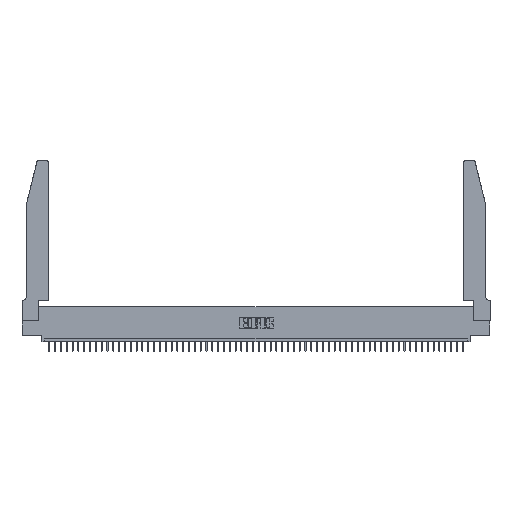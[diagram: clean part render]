
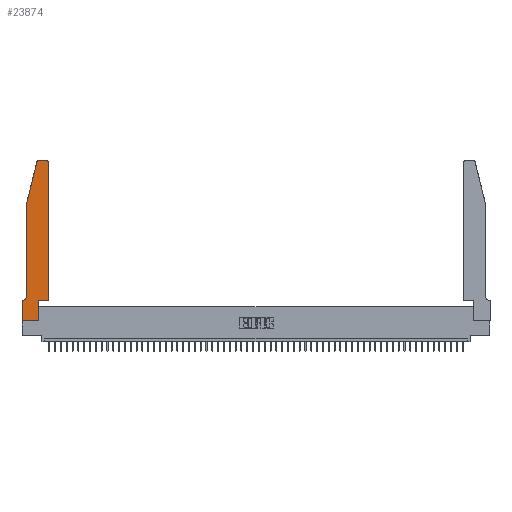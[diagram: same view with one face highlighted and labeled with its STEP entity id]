
A CAD part, top view. The second image highlights one B-rep face of the part: STEP entity #23874.
In plain terms, the highlighted planar face has unit normal (0, 0, 1).
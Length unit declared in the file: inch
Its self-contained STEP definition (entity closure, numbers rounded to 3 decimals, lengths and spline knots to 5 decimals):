
#8 = CARTESIAN_POINT ( 'NONE',  ( 0., 0., 0.37 ) ) ;
#632 = DIRECTION ( 'NONE',  ( 0., -1., 0. ) ) ;
#874 = VERTEX_POINT ( 'NONE', #8 ) ;
#1031 = CARTESIAN_POINT ( 'NONE',  ( 0.4205, 2.72, 0.37 ) ) ;
#1064 = CARTESIAN_POINT ( 'NONE',  ( 0.4505, 0.35, 0.37 ) ) ;
#1419 = DIRECTION ( 'NONE',  ( 1., 0., 0. ) ) ;
#1506 = EDGE_CURVE ( 'NONE', #2203, #23633, #31375, .T. ) ;
#1943 = CARTESIAN_POINT ( 'NONE',  ( 0., 0.35, 0.37 ) ) ;
#2203 = VERTEX_POINT ( 'NONE', #18663 ) ;
#3022 = CARTESIAN_POINT ( 'NONE',  ( 0.2605, 2.75, 0.37 ) ) ;
#3023 = EDGE_CURVE ( 'NONE', #51019, #29257, #23294, .T. ) ;
#3100 = VECTOR ( 'NONE', #11801, 39.37008 ) ;
#3236 = LINE ( 'NONE', #37587, #18646 ) ;
#3475 = DIRECTION ( 'NONE',  ( 0., -1., 0. ) ) ;
#4012 = VECTOR ( 'NONE', #26580, 39.37008 ) ;
#4099 = CARTESIAN_POINT ( 'NONE',  ( 0.0755, 0.42, 0.37 ) ) ;
#4101 = ORIENTED_EDGE ( 'NONE', *, *, #3023, .T. ) ;
#4741 = CARTESIAN_POINT ( 'NONE',  ( 0.0755, 2., 0.37 ) ) ;
#5509 = CIRCLE ( 'NONE', #22926, 0.03 ) ;
#5927 = ORIENTED_EDGE ( 'NONE', *, *, #1506, .T. ) ;
#6037 = ORIENTED_EDGE ( 'NONE', *, *, #28399, .T. ) ;
#7536 = ORIENTED_EDGE ( 'NONE', *, *, #28346, .T. ) ;
#7662 = ORIENTED_EDGE ( 'NONE', *, *, #44084, .T. ) ;
#7664 = AXIS2_PLACEMENT_3D ( 'NONE', #32904, #45919, #41239 ) ;
#10258 = VECTOR ( 'NONE', #23822, 39.37008 ) ;
#10265 = CARTESIAN_POINT ( 'NONE',  ( 0.4505, 2.72, 0.37 ) ) ;
#10451 = LINE ( 'NONE', #45047, #23132 ) ;
#11138 = EDGE_CURVE ( 'NONE', #35823, #874, #10451, .T. ) ;
#11801 = DIRECTION ( 'NONE',  ( -1., 0., 0. ) ) ;
#12817 = LINE ( 'NONE', #3022, #3100 ) ;
#15288 = CARTESIAN_POINT ( 'NONE',  ( 0.4505, 0.35, 0.37 ) ) ;
#15448 = ORIENTED_EDGE ( 'NONE', *, *, #22635, .T. ) ;
#15678 = VERTEX_POINT ( 'NONE', #18632 ) ;
#15884 = EDGE_CURVE ( 'NONE', #30768, #29583, #3236, .T. ) ;
#17616 = DIRECTION ( 'NONE',  ( 0., 0., 1. ) ) ;
#18015 = CARTESIAN_POINT ( 'NONE',  ( 0.2865, 0.35, 0.37 ) ) ;
#18097 = CARTESIAN_POINT ( 'NONE',  ( 0.0055, 0.42, 0.37 ) ) ;
#18213 = FACE_OUTER_BOUND ( 'NONE', #34256, .T. ) ;
#18632 = CARTESIAN_POINT ( 'NONE',  ( 0.284, 2.75, 0.37 ) ) ;
#18646 = VECTOR ( 'NONE', #29566, 39.37008 ) ;
#18663 = CARTESIAN_POINT ( 'NONE',  ( 0.25487, 2.72718, 0.37 ) ) ;
#20030 = DIRECTION ( 'NONE',  ( -1., 0., 0. ) ) ;
#22182 = DIRECTION ( 'NONE',  ( 0., 1., 0. ) ) ;
#22635 = EDGE_CURVE ( 'NONE', #41573, #15678, #12817, .T. ) ;
#22926 = AXIS2_PLACEMENT_3D ( 'NONE', #1031, #17616, #43291 ) ;
#23132 = VECTOR ( 'NONE', #3475, 39.37008 ) ;
#23152 = CARTESIAN_POINT ( 'NONE',  ( 0.2865, 0., 0.37 ) ) ;
#23294 = CIRCLE ( 'NONE', #39969, 0.07 ) ;
#23633 = VERTEX_POINT ( 'NONE', #48153 ) ;
#23822 = DIRECTION ( 'NONE',  ( 1., 0., 0. ) ) ;
#23874 = ADVANCED_FACE ( 'NONE', ( #18213 ), #33083, .T. ) ;
#24409 = VERTEX_POINT ( 'NONE', #1064 ) ;
#26524 = CARTESIAN_POINT ( 'NONE',  ( 0.284, 2.72, 0.37 ) ) ;
#26580 = DIRECTION ( 'NONE',  ( -0.239, -0.971, 0. ) ) ;
#26938 = CARTESIAN_POINT ( 'NONE',  ( 0., 0., 0.37 ) ) ;
#27731 = VECTOR ( 'NONE', #632, 39.37008 ) ;
#28176 = VECTOR ( 'NONE', #1419, 39.37008 ) ;
#28346 = EDGE_CURVE ( 'NONE', #23633, #51019, #42369, .T. ) ;
#28399 = EDGE_CURVE ( 'NONE', #15678, #2203, #38373, .T. ) ;
#29257 = VERTEX_POINT ( 'NONE', #45595 ) ;
#29566 = DIRECTION ( 'NONE',  ( 0., 1., 0. ) ) ;
#29583 = VERTEX_POINT ( 'NONE', #18015 ) ;
#30074 = EDGE_CURVE ( 'NONE', #874, #30768, #41529, .T. ) ;
#30249 = LINE ( 'NONE', #15288, #10258 ) ;
#30768 = VERTEX_POINT ( 'NONE', #23152 ) ;
#31375 = LINE ( 'NONE', #4741, #4012 ) ;
#32351 = VECTOR ( 'NONE', #20030, 39.37008 ) ;
#32904 = CARTESIAN_POINT ( 'NONE',  ( 0., 0.35, 0.37 ) ) ;
#33083 = PLANE ( 'NONE',  #7664 ) ;
#33196 = VECTOR ( 'NONE', #22182, 39.37008 ) ;
#33669 = EDGE_CURVE ( 'NONE', #24409, #47160, #50451, .T. ) ;
#34256 = EDGE_LOOP ( 'NONE', ( #15448, #6037, #5927, #7536, #4101, #42501, #44047, #46259, #50774, #47262, #44667, #7662 ) ) ;
#35073 = DIRECTION ( 'NONE',  ( -1., 0., 0. ) ) ;
#35097 = DIRECTION ( 'NONE',  ( 0., 0., 1. ) ) ;
#35823 = VERTEX_POINT ( 'NONE', #1943 ) ;
#36203 = CARTESIAN_POINT ( 'NONE',  ( 0.0755, 2., 0.37 ) ) ;
#36959 = CARTESIAN_POINT ( 'NONE',  ( 0.0755, 0.35, 0.37 ) ) ;
#37587 = CARTESIAN_POINT ( 'NONE',  ( 0.2865, 0.35, 0.37 ) ) ;
#38373 = CIRCLE ( 'NONE', #46359, 0.03 ) ;
#38839 = EDGE_CURVE ( 'NONE', #29257, #35823, #52945, .T. ) ;
#39969 = AXIS2_PLACEMENT_3D ( 'NONE', #18097, #47144, #35073 ) ;
#41239 = DIRECTION ( 'NONE',  ( 1., 0., 0. ) ) ;
#41529 = LINE ( 'NONE', #26938, #28176 ) ;
#41573 = VERTEX_POINT ( 'NONE', #51893 ) ;
#42369 = LINE ( 'NONE', #36203, #27731 ) ;
#42501 = ORIENTED_EDGE ( 'NONE', *, *, #38839, .T. ) ;
#43291 = DIRECTION ( 'NONE',  ( 1., 0., 0. ) ) ;
#44047 = ORIENTED_EDGE ( 'NONE', *, *, #11138, .T. ) ;
#44084 = EDGE_CURVE ( 'NONE', #47160, #41573, #5509, .T. ) ;
#44397 = DIRECTION ( 'NONE',  ( 1., 0., 0. ) ) ;
#44667 = ORIENTED_EDGE ( 'NONE', *, *, #33669, .T. ) ;
#45047 = CARTESIAN_POINT ( 'NONE',  ( 0., 0., 0.37 ) ) ;
#45595 = CARTESIAN_POINT ( 'NONE',  ( 0.0055, 0.35, 0.37 ) ) ;
#45919 = DIRECTION ( 'NONE',  ( 0., 0., 1. ) ) ;
#46259 = ORIENTED_EDGE ( 'NONE', *, *, #30074, .T. ) ;
#46359 = AXIS2_PLACEMENT_3D ( 'NONE', #26524, #35097, #44397 ) ;
#47144 = DIRECTION ( 'NONE',  ( 0., 0., -1. ) ) ;
#47160 = VERTEX_POINT ( 'NONE', #10265 ) ;
#47262 = ORIENTED_EDGE ( 'NONE', *, *, #48620, .T. ) ;
#48153 = CARTESIAN_POINT ( 'NONE',  ( 0.0755, 2., 0.37 ) ) ;
#48620 = EDGE_CURVE ( 'NONE', #29583, #24409, #30249, .T. ) ;
#50451 = LINE ( 'NONE', #52112, #33196 ) ;
#50774 = ORIENTED_EDGE ( 'NONE', *, *, #15884, .T. ) ;
#51019 = VERTEX_POINT ( 'NONE', #4099 ) ;
#51893 = CARTESIAN_POINT ( 'NONE',  ( 0.4205, 2.75, 0.37 ) ) ;
#52112 = CARTESIAN_POINT ( 'NONE',  ( 0.4505, 0.35, 0.37 ) ) ;
#52945 = LINE ( 'NONE', #36959, #32351 ) ;
